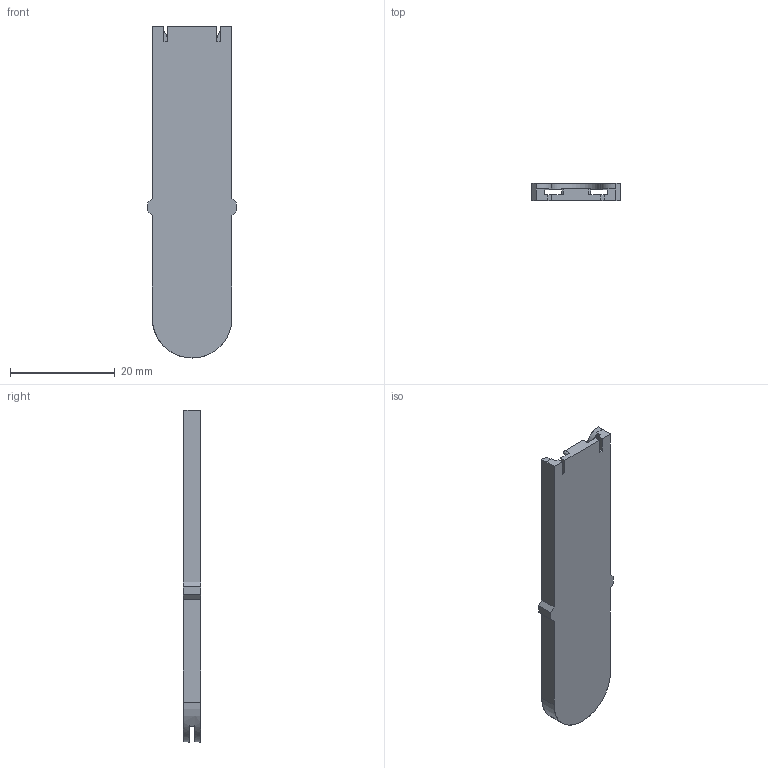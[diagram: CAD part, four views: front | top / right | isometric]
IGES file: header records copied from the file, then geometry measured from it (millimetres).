
Start section: SolidWorks IGES file using analytic representation for surfaces
Global section: file name: SKS5shotclip.IGS; native system: SolidWorks 2013; preprocessor: SolidWorks 2013; author: Greg; date: 130826.092548; units: inch
Bounding box: 16.89 x 3.33 x 63.5 mm (x, y, z)
Surface area: 3052.5 mm2 (no closed solid volume)
Topology: 0 solids, 0 shells, 38 faces, 356 edges, 356 vertices
Faces by surface type: bspline 31, revolution 7
